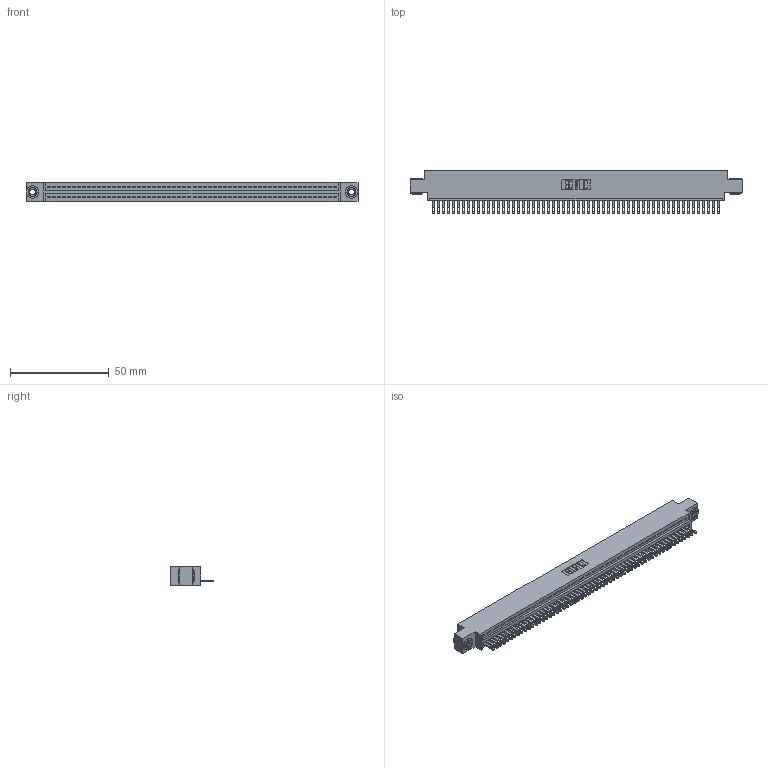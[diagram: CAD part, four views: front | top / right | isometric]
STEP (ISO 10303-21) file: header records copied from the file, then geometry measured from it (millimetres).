
FILE_DESCRIPTION (( 'STEP AP203' ), '1' );
FILE_NAME ('895-058-500-603.STEP', '2020-09-28T02:49:14', ( '' ), ( '' ), 'SwSTEP 2.0', 'SolidWorks 2020', '' );
FILE_SCHEMA (( 'CONFIG_CONTROL_DESIGN' ));
Length unit declared in the file: inch
Products named in the file (4): 845 Part_0.170 Offset - 0.156 Dia-TH; 345-292-001_345-293-100; 895-058-500-603; 345-250-002_345-250-002-102
Assembly tree (61 placements, depth 2):
  895-058-500-603
    845 Part_0.170 Offset - 0.156 Dia-TH
    345-292-001_345-293-100  x58
    345-250-002_345-250-002-102  x2
Bounding box: 168.53 x 21.51 x 9.4 mm (x, y, z)
Volume: 16080 mm3; surface area: 22057.6 mm2
Topology: 61 solids, 61 shells, 3300 faces, 10173 edges, 6778 vertices
Faces by surface type: plane 2066, cylinder 1226, cone 8
Entity records: 42210 total; most frequent: CARTESIAN_POINT 7289, ORIENTED_EDGE 7274, DIRECTION 6375, EDGE_CURVE 3637, LINE 3245, VECTOR 3245, VERTEX_POINT 2422, AXIS2_PLACEMENT_3D 1565
